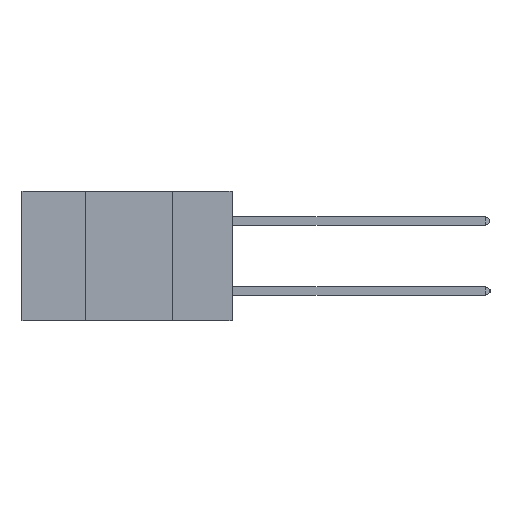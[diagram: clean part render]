
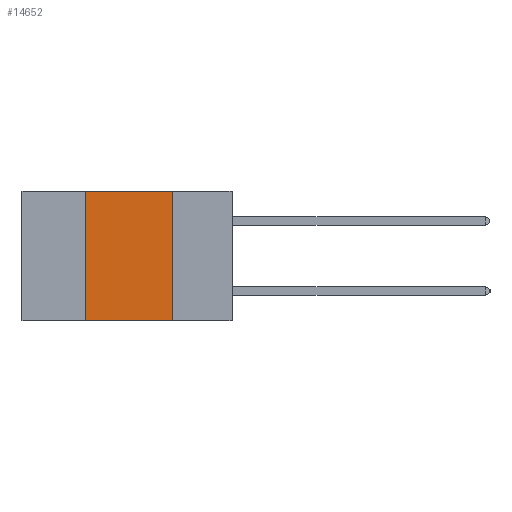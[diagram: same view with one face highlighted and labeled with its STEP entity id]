
A CAD part, left-side view. The second image highlights one B-rep face of the part: STEP entity #14652.
In plain terms, the highlighted planar face has unit normal (-1, 0, 0).
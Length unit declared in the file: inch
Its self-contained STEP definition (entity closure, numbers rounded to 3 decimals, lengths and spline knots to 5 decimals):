
#2442 = VERTEX_POINT ( 'NONE', #18821 ) ;
#3950 = VECTOR ( 'NONE', #15251, 39.37008 ) ;
#4341 = VERTEX_POINT ( 'NONE', #5145 ) ;
#4874 = FACE_OUTER_BOUND ( 'NONE', #12787, .T. ) ;
#5145 = CARTESIAN_POINT ( 'NONE',  ( 0., 0.17, 0. ) ) ;
#5155 = CARTESIAN_POINT ( 'NONE',  ( 0., 0.6, 0. ) ) ;
#6579 = DIRECTION ( 'NONE',  ( 1., 0., 0. ) ) ;
#7411 = VERTEX_POINT ( 'NONE', #20412 ) ;
#7501 = ORIENTED_EDGE ( 'NONE', *, *, #11010, .T. ) ;
#7760 = DIRECTION ( 'NONE',  ( 0., 0., -1. ) ) ;
#8129 = CARTESIAN_POINT ( 'NONE',  ( 0., 0.6, -0.37 ) ) ;
#8343 = LINE ( 'NONE', #5155, #3950 ) ;
#8718 = VERTEX_POINT ( 'NONE', #21634 ) ;
#8783 = EDGE_CURVE ( 'NONE', #2442, #4341, #8343, .T. ) ;
#9240 = LINE ( 'NONE', #8129, #17544 ) ;
#9879 = DIRECTION ( 'NONE',  ( 0., -1., 0. ) ) ;
#9978 = PLANE ( 'NONE',  #19905 ) ;
#10876 = EDGE_CURVE ( 'NONE', #4341, #7411, #16587, .T. ) ;
#10974 = EDGE_CURVE ( 'NONE', #8718, #2442, #19081, .T. ) ;
#10998 = ORIENTED_EDGE ( 'NONE', *, *, #10974, .F. ) ;
#11010 = EDGE_CURVE ( 'NONE', #8718, #7411, #9240, .T. ) ;
#12216 = VECTOR ( 'NONE', #7760, 39.37008 ) ;
#12787 = EDGE_LOOP ( 'NONE', ( #18729, #19258, #10998, #7501 ) ) ;
#14473 = CARTESIAN_POINT ( 'NONE',  ( 0., 0.17, 0. ) ) ;
#14652 = ADVANCED_FACE ( 'NONE', ( #4874 ), #9978, .F. ) ;
#14702 = VECTOR ( 'NONE', #18000, 39.37008 ) ;
#15251 = DIRECTION ( 'NONE',  ( 0., -1., 0. ) ) ;
#16325 = CARTESIAN_POINT ( 'NONE',  ( 0., 0.42, 0. ) ) ;
#16587 = LINE ( 'NONE', #14473, #12216 ) ;
#16616 = CARTESIAN_POINT ( 'NONE',  ( 0., 0.6, 0. ) ) ;
#17544 = VECTOR ( 'NONE', #9879, 39.37008 ) ;
#18000 = DIRECTION ( 'NONE',  ( 0., 0., 1. ) ) ;
#18296 = DIRECTION ( 'NONE',  ( 0., 0., -1. ) ) ;
#18729 = ORIENTED_EDGE ( 'NONE', *, *, #10876, .F. ) ;
#18821 = CARTESIAN_POINT ( 'NONE',  ( 0., 0.42, 0. ) ) ;
#19081 = LINE ( 'NONE', #16325, #14702 ) ;
#19258 = ORIENTED_EDGE ( 'NONE', *, *, #8783, .F. ) ;
#19905 = AXIS2_PLACEMENT_3D ( 'NONE', #16616, #6579, #18296 ) ;
#20412 = CARTESIAN_POINT ( 'NONE',  ( 0., 0.17, -0.37 ) ) ;
#21634 = CARTESIAN_POINT ( 'NONE',  ( 0., 0.42, -0.37 ) ) ;
